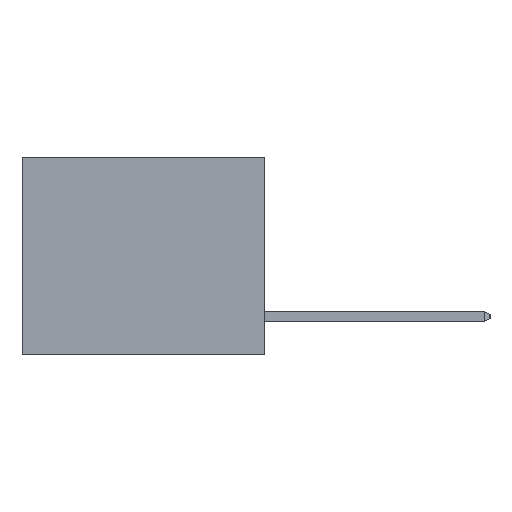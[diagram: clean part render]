
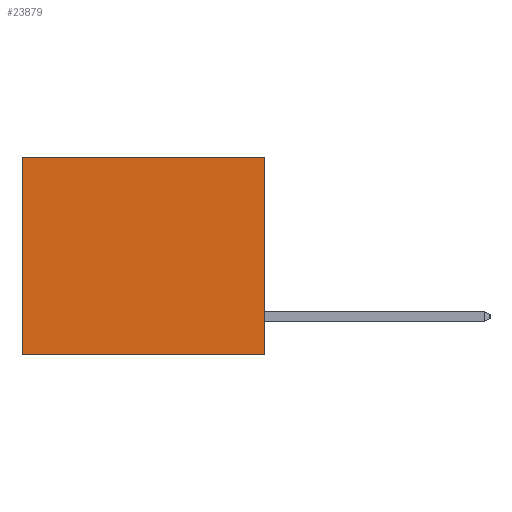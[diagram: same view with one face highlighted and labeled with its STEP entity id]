
A CAD part, left-side view. The second image highlights one B-rep face of the part: STEP entity #23879.
In plain terms, the highlighted planar face has unit normal (-1, 0, 0).
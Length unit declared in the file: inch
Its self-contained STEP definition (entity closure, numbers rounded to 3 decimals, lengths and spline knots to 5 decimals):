
#85 = EDGE_CURVE ( 'NONE', #2980, #1658, #8744, .T. ) ;
#902 = EDGE_CURVE ( 'NONE', #25713, #24882, #10527, .T. ) ;
#996 = DIRECTION ( 'NONE',  ( 0., 0., -1. ) ) ;
#1331 = VECTOR ( 'NONE', #28154, 39.37008 ) ;
#1658 = VERTEX_POINT ( 'NONE', #21246 ) ;
#2632 = FACE_OUTER_BOUND ( 'NONE', #2943, .T. ) ;
#2943 = EDGE_LOOP ( 'NONE', ( #21458, #23916, #14668, #22345 ) ) ;
#2980 = VERTEX_POINT ( 'NONE', #8888 ) ;
#5362 = VECTOR ( 'NONE', #27660, 39.37008 ) ;
#6431 = EDGE_CURVE ( 'NONE', #25713, #2980, #6441, .T. ) ;
#6441 = LINE ( 'NONE', #15185, #29833 ) ;
#7487 = AXIS2_PLACEMENT_3D ( 'NONE', #20174, #12854, #996 ) ;
#8665 = CARTESIAN_POINT ( 'NONE',  ( 0.3165, 0., 0. ) ) ;
#8744 = LINE ( 'NONE', #16168, #1331 ) ;
#8888 = CARTESIAN_POINT ( 'NONE',  ( 0.3165, 0., -0.49 ) ) ;
#10527 = LINE ( 'NONE', #8665, #5362 ) ;
#10979 = DIRECTION ( 'NONE',  ( 0., 0., -1. ) ) ;
#12854 = DIRECTION ( 'NONE',  ( 1., 0., 0. ) ) ;
#14668 = ORIENTED_EDGE ( 'NONE', *, *, #6431, .F. ) ;
#15185 = CARTESIAN_POINT ( 'NONE',  ( 0.3165, 0., -0.49 ) ) ;
#16168 = CARTESIAN_POINT ( 'NONE',  ( 0.3165, 0., -0.49 ) ) ;
#19982 = PLANE ( 'NONE',  #7487 ) ;
#20174 = CARTESIAN_POINT ( 'NONE',  ( 0.3165, 0., -0.49 ) ) ;
#21246 = CARTESIAN_POINT ( 'NONE',  ( 0.3165, 0.6, -0.49 ) ) ;
#21458 = ORIENTED_EDGE ( 'NONE', *, *, #29824, .T. ) ;
#22345 = ORIENTED_EDGE ( 'NONE', *, *, #902, .T. ) ;
#22526 = CARTESIAN_POINT ( 'NONE',  ( 0.3165, 0.6, -0.49 ) ) ;
#23294 = LINE ( 'NONE', #22526, #30674 ) ;
#23741 = CARTESIAN_POINT ( 'NONE',  ( 0.3165, 0.6, 0. ) ) ;
#23879 = ADVANCED_FACE ( 'NONE', ( #2632 ), #19982, .F. ) ;
#23916 = ORIENTED_EDGE ( 'NONE', *, *, #85, .F. ) ;
#24882 = VERTEX_POINT ( 'NONE', #23741 ) ;
#25713 = VERTEX_POINT ( 'NONE', #30144 ) ;
#26765 = DIRECTION ( 'NONE',  ( 0., 0., -1. ) ) ;
#27660 = DIRECTION ( 'NONE',  ( 0., 1., 0. ) ) ;
#28154 = DIRECTION ( 'NONE',  ( 0., 1., 0. ) ) ;
#29824 = EDGE_CURVE ( 'NONE', #24882, #1658, #23294, .T. ) ;
#29833 = VECTOR ( 'NONE', #26765, 39.37008 ) ;
#30144 = CARTESIAN_POINT ( 'NONE',  ( 0.3165, 0., 0. ) ) ;
#30674 = VECTOR ( 'NONE', #10979, 39.37008 ) ;
